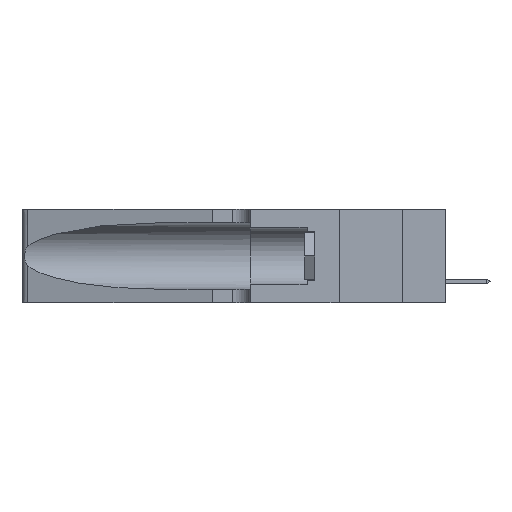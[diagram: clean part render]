
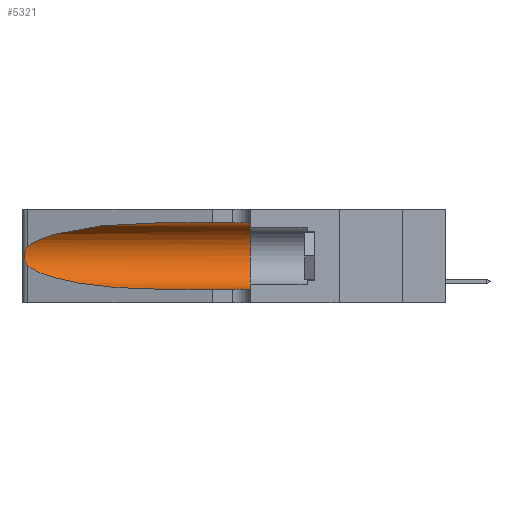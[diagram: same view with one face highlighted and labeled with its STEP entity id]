
A CAD part, left-side view. The second image highlights one B-rep face of the part: STEP entity #5321.
In plain terms, the highlighted cylindrical face has radius 3.308 mm (diameter 6.617 mm), a partial arc.
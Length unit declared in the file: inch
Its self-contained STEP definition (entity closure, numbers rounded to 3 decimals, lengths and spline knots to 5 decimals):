
#964 = VERTEX_POINT ( 'NONE', #21105 ) ;
#1516 = CARTESIAN_POINT ( 'NONE',  ( 0.26017, 1.23833, 0.17102 ) ) ;
#2375 = LINE ( 'NONE', #22953, #31496 ) ;
#2621 = B_SPLINE_CURVE_WITH_KNOTS ( 'NONE', 3,
 ( #8513, #7702, #20604, #5365, #32570, #8617, #14554, #16479, #1516, #22587, #13778, #17328, #25581, #7560 ),
 .UNSPECIFIED., .F., .F.,
 ( 4, 2, 2, 2, 2, 2, 4 ),
 ( 0., 0.00027, 0.00053, 0.00107, 0.0016, 0.00187, 0.00214 ),
 .UNSPECIFIED. ) ;
#2734 = VERTEX_POINT ( 'NONE', #13471 ) ;
#2837 = AXIS2_PLACEMENT_3D ( 'NONE', #13588, #16559, #28852 ) ;
#3701 = CARTESIAN_POINT ( 'NONE',  ( 0.25487, 1.22718, 0.22369 ) ) ;
#3834 = CARTESIAN_POINT ( 'NONE',  ( 0.2373, 1.15595, 0.28018 ) ) ;
#5321 = ADVANCED_FACE ( 'NONE', ( #24045 ), #32088, .F. ) ;
#5326 = ORIENTED_EDGE ( 'NONE', *, *, #21059, .F. ) ;
#5365 = CARTESIAN_POINT ( 'NONE',  ( 0.25787, 1.23484, 0.2124 ) ) ;
#5957 = AXIS2_PLACEMENT_3D ( 'NONE', #31143, #16123, #6385 ) ;
#6385 = DIRECTION ( 'NONE',  ( 0., 0., 1. ) ) ;
#6772 = VERTEX_POINT ( 'NONE', #28628 ) ;
#7203 = CIRCLE ( 'NONE', #5957, 0.13025 ) ;
#7560 = CARTESIAN_POINT ( 'NONE',  ( 0.25487, 1.22718, 0.14631 ) ) ;
#7702 = CARTESIAN_POINT ( 'NONE',  ( 0.25555, 1.22994, 0.2215 ) ) ;
#8088 = VECTOR ( 'NONE', #23206, 39.37008 ) ;
#8513 = CARTESIAN_POINT ( 'NONE',  ( 0.25487, 1.22718, 0.22369 ) ) ;
#8617 = CARTESIAN_POINT ( 'NONE',  ( 0.26018, 1.23835, 0.19895 ) ) ;
#9599 = CARTESIAN_POINT ( 'NONE',  ( 0.1305, 0.72297, 0.31525 ) ) ;
#10498 = CARTESIAN_POINT ( 'NONE',  ( 0.1305, 0.35, 0.31525 ) ) ;
#11996 =( BOUNDED_CURVE ( )  B_SPLINE_CURVE ( 3, ( #24343, #13068, #27905, #21987 ),
 .UNSPECIFIED., .F., .F. ) 
 B_SPLINE_CURVE_WITH_KNOTS ( ( 4, 4 ),
 ( 3.44316, 4.71239 ),
 .UNSPECIFIED. ) 
 CURVE ( )  GEOMETRIC_REPRESENTATION_ITEM ( )  RATIONAL_B_SPLINE_CURVE ( ( 1., 0.87, 0.87, 1. ) ) 
 REPRESENTATION_ITEM ( '' )  );
#12177 = EDGE_CURVE ( 'NONE', #15008, #6772, #32934, .T. ) ;
#12385 = CARTESIAN_POINT ( 'NONE',  ( 0.18966, 0.96281, 0.31525 ) ) ;
#13068 = CARTESIAN_POINT ( 'NONE',  ( 0.2373, 1.15595, 0.08982 ) ) ;
#13471 = CARTESIAN_POINT ( 'NONE',  ( 0.25487, 1.22718, 0.14631 ) ) ;
#13588 = CARTESIAN_POINT ( 'NONE',  ( 0.1305, 1.61858, 0.185 ) ) ;
#13778 = CARTESIAN_POINT ( 'NONE',  ( 0.25789, 1.23486, 0.15765 ) ) ;
#14245 = CARTESIAN_POINT ( 'NONE',  ( 0.1305, 1.61858, 0.31525 ) ) ;
#14324 = EDGE_LOOP ( 'NONE', ( #18321, #28343, #19619, #35476, #25968, #5326 ) ) ;
#14554 = CARTESIAN_POINT ( 'NONE',  ( 0.26075, 1.23896, 0.19203 ) ) ;
#15008 = VERTEX_POINT ( 'NONE', #36478 ) ;
#16123 = DIRECTION ( 'NONE',  ( 0., 1., 0. ) ) ;
#16479 = CARTESIAN_POINT ( 'NONE',  ( 0.26075, 1.23896, 0.178 ) ) ;
#16559 = DIRECTION ( 'NONE',  ( 0., -1., 0. ) ) ;
#17328 = CARTESIAN_POINT ( 'NONE',  ( 0.25639, 1.23186, 0.15144 ) ) ;
#18321 = ORIENTED_EDGE ( 'NONE', *, *, #12177, .T. ) ;
#19619 = ORIENTED_EDGE ( 'NONE', *, *, #31481, .T. ) ;
#19848 = EDGE_CURVE ( 'NONE', #6772, #2734, #2621, .T. ) ;
#20604 = CARTESIAN_POINT ( 'NONE',  ( 0.25639, 1.23184, 0.21858 ) ) ;
#21059 = EDGE_CURVE ( 'NONE', #15008, #23877, #24054, .T. ) ;
#21105 = CARTESIAN_POINT ( 'NONE',  ( 0.1305, 0.72297, 0.05475 ) ) ;
#21987 = CARTESIAN_POINT ( 'NONE',  ( 0.1305, 0.72297, 0.05475 ) ) ;
#22587 = CARTESIAN_POINT ( 'NONE',  ( 0.25856, 1.23593, 0.16098 ) ) ;
#22953 = CARTESIAN_POINT ( 'NONE',  ( 0.1305, 1.61858, 0.05475 ) ) ;
#23206 = DIRECTION ( 'NONE',  ( 0., -1., 0. ) ) ;
#23877 = VERTEX_POINT ( 'NONE', #10498 ) ;
#24045 = FACE_OUTER_BOUND ( 'NONE', #14324, .T. ) ;
#24054 = LINE ( 'NONE', #14245, #8088 ) ;
#24236 = VERTEX_POINT ( 'NONE', #27030 ) ;
#24343 = CARTESIAN_POINT ( 'NONE',  ( 0.25487, 1.22718, 0.14631 ) ) ;
#25581 = CARTESIAN_POINT ( 'NONE',  ( 0.25555, 1.22993, 0.14849 ) ) ;
#25822 = DIRECTION ( 'NONE',  ( 0., -1., 0. ) ) ;
#25968 = ORIENTED_EDGE ( 'NONE', *, *, #26446, .F. ) ;
#26446 = EDGE_CURVE ( 'NONE', #23877, #24236, #7203, .T. ) ;
#27030 = CARTESIAN_POINT ( 'NONE',  ( 0.1305, 0.35, 0.05475 ) ) ;
#27905 = CARTESIAN_POINT ( 'NONE',  ( 0.18966, 0.96281, 0.05475 ) ) ;
#28343 = ORIENTED_EDGE ( 'NONE', *, *, #19848, .T. ) ;
#28628 = CARTESIAN_POINT ( 'NONE',  ( 0.25487, 1.22718, 0.22369 ) ) ;
#28852 = DIRECTION ( 'NONE',  ( 0., 0., -1. ) ) ;
#31143 = CARTESIAN_POINT ( 'NONE',  ( 0.1305, 0.35, 0.185 ) ) ;
#31481 = EDGE_CURVE ( 'NONE', #2734, #964, #11996, .T. ) ;
#31496 = VECTOR ( 'NONE', #25822, 39.37008 ) ;
#32088 = CYLINDRICAL_SURFACE ( 'NONE', #2837, 0.13025 ) ;
#32570 = CARTESIAN_POINT ( 'NONE',  ( 0.25854, 1.2359, 0.20912 ) ) ;
#32934 =( BOUNDED_CURVE ( )  B_SPLINE_CURVE ( 3, ( #9599, #12385, #3834, #3701 ),
 .UNSPECIFIED., .F., .F. ) 
 B_SPLINE_CURVE_WITH_KNOTS ( ( 4, 4 ),
 ( 1.5708, 2.84003 ),
 .UNSPECIFIED. ) 
 CURVE ( )  GEOMETRIC_REPRESENTATION_ITEM ( )  RATIONAL_B_SPLINE_CURVE ( ( 1., 0.87, 0.87, 1. ) ) 
 REPRESENTATION_ITEM ( '' )  );
#32960 = EDGE_CURVE ( 'NONE', #964, #24236, #2375, .T. ) ;
#35476 = ORIENTED_EDGE ( 'NONE', *, *, #32960, .T. ) ;
#36478 = CARTESIAN_POINT ( 'NONE',  ( 0.1305, 0.72297, 0.31525 ) ) ;
